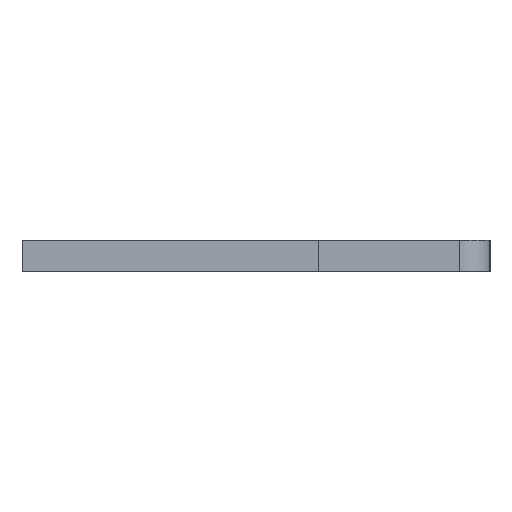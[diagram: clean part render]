
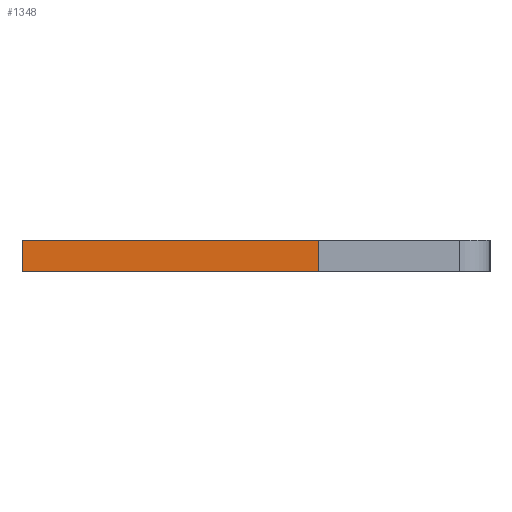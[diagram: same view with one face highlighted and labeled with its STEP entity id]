
A CAD part, left-side view. The second image highlights one B-rep face of the part: STEP entity #1348.
In plain terms, the highlighted face is planar.
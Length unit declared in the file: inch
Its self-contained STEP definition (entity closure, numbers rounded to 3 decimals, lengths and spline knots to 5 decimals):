
#81 = DIRECTION ( 'NONE',  ( 0., 1., 0. ) ) ;
#84 = CARTESIAN_POINT ( 'NONE',  ( 0.01, 0.15, -0.04 ) ) ;
#120 = VECTOR ( 'NONE', #768, 39.37008 ) ;
#148 = LINE ( 'NONE', #899, #1047 ) ;
#185 = CARTESIAN_POINT ( 'NONE',  ( 0.01, -0.04, -0.04 ) ) ;
#311 = CARTESIAN_POINT ( 'NONE',  ( 0.01, 0.15, -0.04 ) ) ;
#400 = AXIS2_PLACEMENT_3D ( 'NONE', #555, #563, #567 ) ;
#409 = ORIENTED_EDGE ( 'NONE', *, *, #994, .F. ) ;
#413 = LINE ( 'NONE', #311, #120 ) ;
#434 = CARTESIAN_POINT ( 'NONE',  ( 0.01, 0.15, -0.04 ) ) ;
#454 = CARTESIAN_POINT ( 'NONE',  ( 0.01, -0.04, -0.04 ) ) ;
#555 = CARTESIAN_POINT ( 'NONE',  ( 0.01, 0.15, -0.04 ) ) ;
#563 = DIRECTION ( 'NONE',  ( 0., 0., 1. ) ) ;
#567 = DIRECTION ( 'NONE',  ( 1., 0., 0. ) ) ;
#594 = EDGE_LOOP ( 'NONE', ( #775, #409, #1441, #705 ) ) ;
#598 = LINE ( 'NONE', #454, #929 ) ;
#657 = VERTEX_POINT ( 'NONE', #185 ) ;
#692 = EDGE_CURVE ( 'NONE', #657, #1149, #968, .T. ) ;
#705 = ORIENTED_EDGE ( 'NONE', *, *, #799, .T. ) ;
#768 = DIRECTION ( 'NONE',  ( -1., 0., 0. ) ) ;
#775 = ORIENTED_EDGE ( 'NONE', *, *, #998, .T. ) ;
#799 = EDGE_CURVE ( 'NONE', #657, #1448, #598, .T. ) ;
#827 = VERTEX_POINT ( 'NONE', #1021 ) ;
#866 = FACE_OUTER_BOUND ( 'NONE', #594, .T. ) ;
#899 = CARTESIAN_POINT ( 'NONE',  ( -0.01, 0.15, -0.04 ) ) ;
#929 = VECTOR ( 'NONE', #1268, 39.37008 ) ;
#968 = LINE ( 'NONE', #84, #1240 ) ;
#994 = EDGE_CURVE ( 'NONE', #1149, #827, #413, .T. ) ;
#998 = EDGE_CURVE ( 'NONE', #1448, #827, #148, .T. ) ;
#1016 = DIRECTION ( 'NONE',  ( 0., 1., 0. ) ) ;
#1021 = CARTESIAN_POINT ( 'NONE',  ( -0.01, 0.15, -0.04 ) ) ;
#1047 = VECTOR ( 'NONE', #1016, 39.37008 ) ;
#1149 = VERTEX_POINT ( 'NONE', #434 ) ;
#1240 = VECTOR ( 'NONE', #81, 39.37008 ) ;
#1268 = DIRECTION ( 'NONE',  ( -1., 0., 0. ) ) ;
#1279 = PLANE ( 'NONE',  #400 ) ;
#1348 = ADVANCED_FACE ( 'NONE', ( #866 ), #1279, .F. ) ;
#1407 = CARTESIAN_POINT ( 'NONE',  ( -0.01, -0.04, -0.04 ) ) ;
#1441 = ORIENTED_EDGE ( 'NONE', *, *, #692, .F. ) ;
#1448 = VERTEX_POINT ( 'NONE', #1407 ) ;
